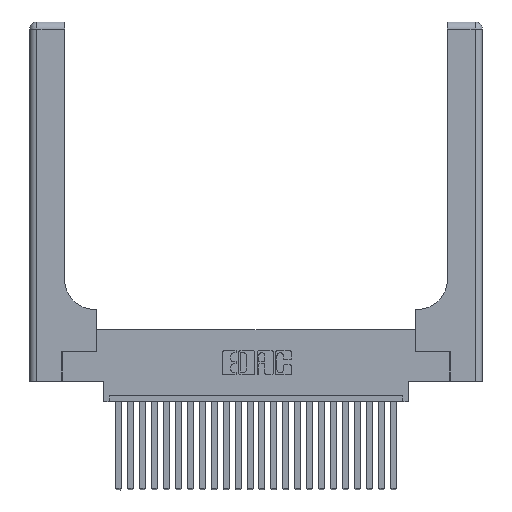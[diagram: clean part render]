
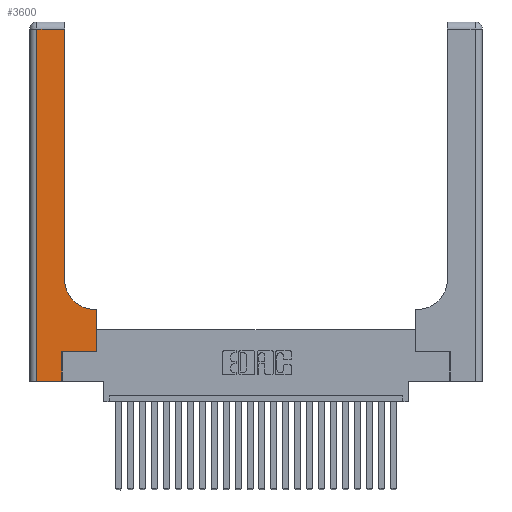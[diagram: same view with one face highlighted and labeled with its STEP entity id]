
A CAD part, top view. The second image highlights one B-rep face of the part: STEP entity #3600.
In plain terms, the highlighted planar face has unit normal (0, 0, 1).
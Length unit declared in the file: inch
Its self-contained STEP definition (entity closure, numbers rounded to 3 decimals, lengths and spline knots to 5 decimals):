
#152 = VECTOR ( 'NONE', #5112, 39.37008 ) ;
#156 = EDGE_CURVE ( 'NONE', #20780, #7737, #10907, .T. ) ;
#389 = VERTEX_POINT ( 'NONE', #17979 ) ;
#1459 = DIRECTION ( 'NONE',  ( 0., -1., 0. ) ) ;
#1680 = EDGE_CURVE ( 'NONE', #389, #12789, #23818, .T. ) ;
#1696 = VECTOR ( 'NONE', #4913, 39.37008 ) ;
#1743 = LINE ( 'NONE', #12980, #3592 ) ;
#2244 = EDGE_CURVE ( 'NONE', #16663, #6617, #8944, .T. ) ;
#3592 = VECTOR ( 'NONE', #24636, 39.37008 ) ;
#3600 = ADVANCED_FACE ( 'NONE', ( #5087 ), #9443, .F. ) ;
#4792 = CARTESIAN_POINT ( 'NONE',  ( 0., 2.94, 0.37 ) ) ;
#4913 = DIRECTION ( 'NONE',  ( 0., 1., 0. ) ) ;
#5087 = FACE_OUTER_BOUND ( 'NONE', #7939, .T. ) ;
#5112 = DIRECTION ( 'NONE',  ( 1., 0., 0. ) ) ;
#5183 = CARTESIAN_POINT ( 'NONE',  ( 0.5415, 0.85, 0.37 ) ) ;
#5290 = CARTESIAN_POINT ( 'NONE',  ( 0.2915, 0.85, 0.37 ) ) ;
#5997 = DIRECTION ( 'NONE',  ( 1., 0., 0. ) ) ;
#6617 = VERTEX_POINT ( 'NONE', #8206 ) ;
#6938 = LINE ( 'NONE', #14520, #1696 ) ;
#7013 = ORIENTED_EDGE ( 'NONE', *, *, #156, .T. ) ;
#7175 = DIRECTION ( 'NONE',  ( 0., 0., -1. ) ) ;
#7349 = LINE ( 'NONE', #7426, #17274 ) ;
#7426 = CARTESIAN_POINT ( 'NONE',  ( 0.06, 3., 0.37 ) ) ;
#7737 = VERTEX_POINT ( 'NONE', #22262 ) ;
#7939 = EDGE_LOOP ( 'NONE', ( #14805, #10882, #14518, #13051, #7013, #15387, #8772, #21659, #17210 ) ) ;
#8048 = VECTOR ( 'NONE', #12799, 39.37008 ) ;
#8206 = CARTESIAN_POINT ( 'NONE',  ( 0.06, 2.94, 0.37 ) ) ;
#8390 = CARTESIAN_POINT ( 'NONE',  ( 0.2915, 2.94, 0.37 ) ) ;
#8607 = CARTESIAN_POINT ( 'NONE',  ( 0.269, 0., 0.37 ) ) ;
#8772 = ORIENTED_EDGE ( 'NONE', *, *, #18610, .T. ) ;
#8944 = LINE ( 'NONE', #4792, #8048 ) ;
#9443 = PLANE ( 'NONE',  #10168 ) ;
#9816 = CARTESIAN_POINT ( 'NONE',  ( 0., 0., 0.37 ) ) ;
#10168 = AXIS2_PLACEMENT_3D ( 'NONE', #21462, #23254, #13512 ) ;
#10277 = VECTOR ( 'NONE', #5997, 39.37008 ) ;
#10882 = ORIENTED_EDGE ( 'NONE', *, *, #2244, .T. ) ;
#10907 = LINE ( 'NONE', #8607, #19901 ) ;
#12469 = CARTESIAN_POINT ( 'NONE',  ( 0.269, 0.25, 0.37 ) ) ;
#12686 = CARTESIAN_POINT ( 'NONE',  ( 0.2915, 0.6, 0.37 ) ) ;
#12789 = VERTEX_POINT ( 'NONE', #25444 ) ;
#12799 = DIRECTION ( 'NONE',  ( -1., 0., 0. ) ) ;
#12980 = CARTESIAN_POINT ( 'NONE',  ( 0.2915, 3., 0.37 ) ) ;
#13051 = ORIENTED_EDGE ( 'NONE', *, *, #19514, .T. ) ;
#13210 = EDGE_CURVE ( 'NONE', #7737, #13806, #25209, .T. ) ;
#13297 = EDGE_CURVE ( 'NONE', #18082, #16663, #1743, .T. ) ;
#13512 = DIRECTION ( 'NONE',  ( -1., 0., 0. ) ) ;
#13806 = VERTEX_POINT ( 'NONE', #22252 ) ;
#14455 = AXIS2_PLACEMENT_3D ( 'NONE', #5183, #7175, #25039 ) ;
#14518 = ORIENTED_EDGE ( 'NONE', *, *, #24922, .T. ) ;
#14520 = CARTESIAN_POINT ( 'NONE',  ( 0.5585, 0.25, 0.37 ) ) ;
#14597 = DIRECTION ( 'NONE',  ( -1., 0., 0. ) ) ;
#14805 = ORIENTED_EDGE ( 'NONE', *, *, #13297, .T. ) ;
#15387 = ORIENTED_EDGE ( 'NONE', *, *, #13210, .T. ) ;
#16663 = VERTEX_POINT ( 'NONE', #8390 ) ;
#16760 = VECTOR ( 'NONE', #14597, 39.37008 ) ;
#17085 = CARTESIAN_POINT ( 'NONE',  ( 0.06, 0., 0.37 ) ) ;
#17210 = ORIENTED_EDGE ( 'NONE', *, *, #22131, .T. ) ;
#17274 = VECTOR ( 'NONE', #1459, 39.37008 ) ;
#17979 = CARTESIAN_POINT ( 'NONE',  ( 0.5585, 0.6, 0.37 ) ) ;
#18082 = VERTEX_POINT ( 'NONE', #5290 ) ;
#18610 = EDGE_CURVE ( 'NONE', #13806, #389, #6938, .T. ) ;
#19514 = EDGE_CURVE ( 'NONE', #21540, #20780, #21443, .T. ) ;
#19901 = VECTOR ( 'NONE', #22462, 39.37008 ) ;
#20780 = VERTEX_POINT ( 'NONE', #22615 ) ;
#20961 = CIRCLE ( 'NONE', #14455, 0.25 ) ;
#21443 = LINE ( 'NONE', #9816, #10277 ) ;
#21462 = CARTESIAN_POINT ( 'NONE',  ( 0., 3., 0.37 ) ) ;
#21540 = VERTEX_POINT ( 'NONE', #17085 ) ;
#21659 = ORIENTED_EDGE ( 'NONE', *, *, #1680, .T. ) ;
#22131 = EDGE_CURVE ( 'NONE', #12789, #18082, #20961, .T. ) ;
#22252 = CARTESIAN_POINT ( 'NONE',  ( 0.5585, 0.25, 0.37 ) ) ;
#22262 = CARTESIAN_POINT ( 'NONE',  ( 0.269, 0.25, 0.37 ) ) ;
#22462 = DIRECTION ( 'NONE',  ( 0., 1., 0. ) ) ;
#22615 = CARTESIAN_POINT ( 'NONE',  ( 0.269, 0., 0.37 ) ) ;
#23254 = DIRECTION ( 'NONE',  ( 0., 0., -1. ) ) ;
#23818 = LINE ( 'NONE', #12686, #16760 ) ;
#24636 = DIRECTION ( 'NONE',  ( 0., 1., 0. ) ) ;
#24922 = EDGE_CURVE ( 'NONE', #6617, #21540, #7349, .T. ) ;
#25039 = DIRECTION ( 'NONE',  ( 1., 0., 0. ) ) ;
#25209 = LINE ( 'NONE', #12469, #152 ) ;
#25444 = CARTESIAN_POINT ( 'NONE',  ( 0.5415, 0.6, 0.37 ) ) ;
